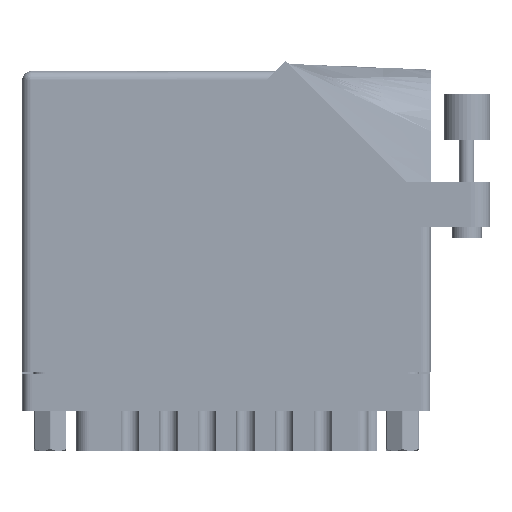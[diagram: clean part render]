
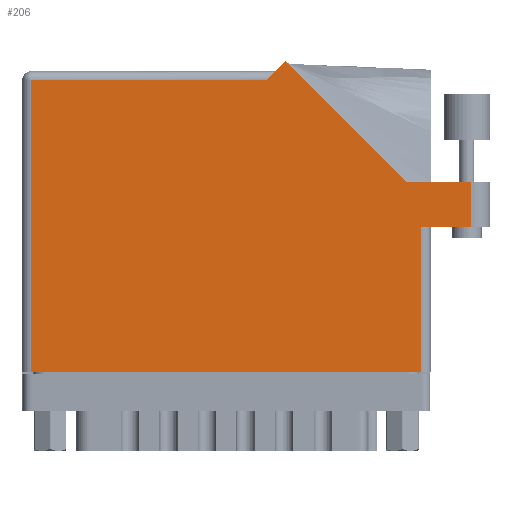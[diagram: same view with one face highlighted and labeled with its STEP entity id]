
A CAD part, front view. The second image highlights one B-rep face of the part: STEP entity #206.
In plain terms, the highlighted face is planar.
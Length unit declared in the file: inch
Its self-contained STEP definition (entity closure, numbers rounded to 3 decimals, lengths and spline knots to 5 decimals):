
#206 = ADVANCED_FACE ( 'NONE', ( #21780 ), #77940, .F. ) ;
#261 = CARTESIAN_POINT ( 'NONE',  ( 2.755, 0.98, 0. ) ) ;
#849 = ORIENTED_EDGE ( 'NONE', *, *, #51670, .T. ) ;
#1199 = LINE ( 'NONE', #97200, #102503 ) ;
#2303 = DIRECTION ( 'NONE',  ( 1., 0., 0. ) ) ;
#2331 = DIRECTION ( 'NONE',  ( 0., 1., 0. ) ) ;
#3211 = EDGE_LOOP ( 'NONE', ( #57958, #103031, #45156, #52806, #849, #86262, #60429, #64079, #83835 ) ) ;
#4151 = CARTESIAN_POINT ( 'NONE',  ( 0.062, 0., 0. ) ) ;
#5117 = VERTEX_POINT ( 'NONE', #33761 ) ;
#5526 = CARTESIAN_POINT ( 'NONE',  ( 1.643, 1.968, 0. ) ) ;
#8577 = EDGE_CURVE ( 'NONE', #37962, #5117, #99092, .T. ) ;
#10386 = DIRECTION ( 'NONE',  ( -0.707, -0.707, 0. ) ) ;
#11751 = CARTESIAN_POINT ( 'NONE',  ( 2.693, 0.98, 0. ) ) ;
#13824 = VECTOR ( 'NONE', #62566, 39.37008 ) ;
#13933 = AXIS2_PLACEMENT_3D ( 'NONE', #79345, #55991, #14817 ) ;
#14817 = DIRECTION ( 'NONE',  ( -1., 0., 0. ) ) ;
#17522 = CARTESIAN_POINT ( 'NONE',  ( 1.705, 2.03, 0. ) ) ;
#17616 = EDGE_CURVE ( 'NONE', #58696, #105160, #53587, .T. ) ;
#18292 = EDGE_CURVE ( 'NONE', #5117, #52684, #72673, .T. ) ;
#19639 = VECTOR ( 'NONE', #2303, 39.37008 ) ;
#21695 = VECTOR ( 'NONE', #71659, 39.37008 ) ;
#21780 = FACE_OUTER_BOUND ( 'NONE', #3211, .T. ) ;
#24708 = LINE ( 'NONE', #261, #72126 ) ;
#26565 = CARTESIAN_POINT ( 'NONE',  ( 3.155, 1.287, 0. ) ) ;
#30853 = EDGE_CURVE ( 'NONE', #100821, #49629, #1199, .T. ) ;
#33518 = DIRECTION ( 'NONE',  ( 1., 0., 0. ) ) ;
#33761 = CARTESIAN_POINT ( 'NONE',  ( 2.693, 0., 0. ) ) ;
#34220 = CARTESIAN_POINT ( 'NONE',  ( 0.062, 0., 0. ) ) ;
#35542 = EDGE_CURVE ( 'NONE', #37102, #79994, #38296, .T. ) ;
#37102 = VERTEX_POINT ( 'NONE', #101732 ) ;
#37962 = VERTEX_POINT ( 'NONE', #4151 ) ;
#38296 = LINE ( 'NONE', #97740, #21695 ) ;
#39496 = LINE ( 'NONE', #17522, #60088 ) ;
#44165 = EDGE_CURVE ( 'NONE', #52684, #100821, #24708, .T. ) ;
#45156 = ORIENTED_EDGE ( 'NONE', *, *, #88215, .T. ) ;
#49629 = VERTEX_POINT ( 'NONE', #53746 ) ;
#51670 = EDGE_CURVE ( 'NONE', #79994, #58696, #39496, .T. ) ;
#51927 = VECTOR ( 'NONE', #74746, 39.37008 ) ;
#52684 = VERTEX_POINT ( 'NONE', #98451 ) ;
#52806 = ORIENTED_EDGE ( 'NONE', *, *, #35542, .T. ) ;
#53587 = LINE ( 'NONE', #54289, #13824 ) ;
#53605 = EDGE_CURVE ( 'NONE', #105160, #37962, #76375, .T. ) ;
#53746 = CARTESIAN_POINT ( 'NONE',  ( 3.03, 1.287, 0. ) ) ;
#54289 = CARTESIAN_POINT ( 'NONE',  ( 0., 1.968, 0. ) ) ;
#55991 = DIRECTION ( 'NONE',  ( 0., 0., -1. ) ) ;
#57958 = ORIENTED_EDGE ( 'NONE', *, *, #44165, .T. ) ;
#58696 = VERTEX_POINT ( 'NONE', #5526 ) ;
#59485 = DIRECTION ( 'NONE',  ( -1., 0., 0. ) ) ;
#59513 = LINE ( 'NONE', #26565, #97943 ) ;
#60088 = VECTOR ( 'NONE', #10386, 39.37008 ) ;
#60429 = ORIENTED_EDGE ( 'NONE', *, *, #53605, .T. ) ;
#62566 = DIRECTION ( 'NONE',  ( -1., 0., 0. ) ) ;
#64079 = ORIENTED_EDGE ( 'NONE', *, *, #8577, .T. ) ;
#66449 = CARTESIAN_POINT ( 'NONE',  ( 0., 0., 0. ) ) ;
#69866 = CARTESIAN_POINT ( 'NONE',  ( 0.062, 1.968, 0. ) ) ;
#71015 = CARTESIAN_POINT ( 'NONE',  ( 3.03, 0.98, 0. ) ) ;
#71659 = DIRECTION ( 'NONE',  ( -0.707, 0.707, 0. ) ) ;
#72126 = VECTOR ( 'NONE', #33518, 39.37008 ) ;
#72673 = LINE ( 'NONE', #11751, #99533 ) ;
#74746 = DIRECTION ( 'NONE',  ( 0., -1., 0. ) ) ;
#76375 = LINE ( 'NONE', #34220, #51927 ) ;
#77940 = PLANE ( 'NONE',  #13933 ) ;
#79345 = CARTESIAN_POINT ( 'NONE',  ( 0., 2.03, 0. ) ) ;
#79994 = VERTEX_POINT ( 'NONE', #104407 ) ;
#81843 = DIRECTION ( 'NONE',  ( 0., 1., 0. ) ) ;
#83835 = ORIENTED_EDGE ( 'NONE', *, *, #18292, .T. ) ;
#86262 = ORIENTED_EDGE ( 'NONE', *, *, #17616, .T. ) ;
#88215 = EDGE_CURVE ( 'NONE', #49629, #37102, #59513, .T. ) ;
#97200 = CARTESIAN_POINT ( 'NONE',  ( 3.03, 1.287, 0. ) ) ;
#97740 = CARTESIAN_POINT ( 'NONE',  ( 2.58942, 1.287, 0. ) ) ;
#97943 = VECTOR ( 'NONE', #59485, 39.37008 ) ;
#98451 = CARTESIAN_POINT ( 'NONE',  ( 2.693, 0.98, 0. ) ) ;
#99092 = LINE ( 'NONE', #66449, #19639 ) ;
#99533 = VECTOR ( 'NONE', #2331, 39.37008 ) ;
#100821 = VERTEX_POINT ( 'NONE', #71015 ) ;
#101732 = CARTESIAN_POINT ( 'NONE',  ( 2.58942, 1.287, 0. ) ) ;
#102503 = VECTOR ( 'NONE', #81843, 39.37008 ) ;
#103031 = ORIENTED_EDGE ( 'NONE', *, *, #30853, .T. ) ;
#104407 = CARTESIAN_POINT ( 'NONE',  ( 1.77571, 2.10071, 0. ) ) ;
#105160 = VERTEX_POINT ( 'NONE', #69866 ) ;
